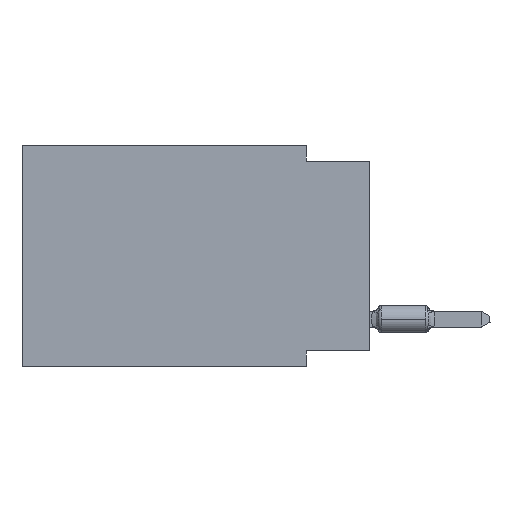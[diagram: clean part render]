
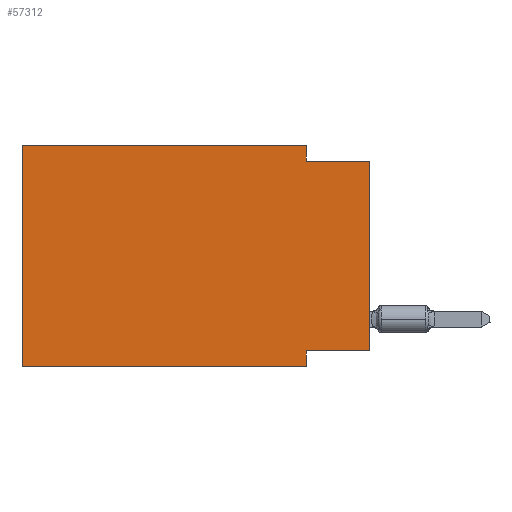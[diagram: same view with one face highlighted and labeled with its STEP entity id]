
A CAD part, left-side view. The second image highlights one B-rep face of the part: STEP entity #57312.
In plain terms, the highlighted planar face has unit normal (-1, 0, 0).
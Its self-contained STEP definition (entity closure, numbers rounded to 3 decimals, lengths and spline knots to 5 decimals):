
#2422 = EDGE_CURVE ( 'NONE', #3368, #60465, #82838, .T. ) ;
#3368 = VERTEX_POINT ( 'NONE', #6891 ) ;
#6891 = CARTESIAN_POINT ( 'NONE',  ( 0., 0.1, -0.325 ) ) ;
#7135 = ORIENTED_EDGE ( 'NONE', *, *, #54907, .F. ) ;
#7476 = DIRECTION ( 'NONE',  ( 0., -1., 0. ) ) ;
#9867 = CARTESIAN_POINT ( 'NONE',  ( 0., 0.55, 0. ) ) ;
#10330 = CARTESIAN_POINT ( 'NONE',  ( 0., 0.55, -0.35 ) ) ;
#13351 = ORIENTED_EDGE ( 'NONE', *, *, #19834, .F. ) ;
#15161 = CARTESIAN_POINT ( 'NONE',  ( 0., 0., -0.025 ) ) ;
#16466 = AXIS2_PLACEMENT_3D ( 'NONE', #69238, #44053, #76487 ) ;
#19517 = CARTESIAN_POINT ( 'NONE',  ( 0., 0.1, 0. ) ) ;
#19834 = EDGE_CURVE ( 'NONE', #46831, #79480, #67953, .T. ) ;
#19960 = LINE ( 'NONE', #65215, #42718 ) ;
#23024 = VERTEX_POINT ( 'NONE', #57015 ) ;
#23394 = ORIENTED_EDGE ( 'NONE', *, *, #31127, .T. ) ;
#23513 = DIRECTION ( 'NONE',  ( 0., 0., -1. ) ) ;
#25919 = LINE ( 'NONE', #19517, #65794 ) ;
#27560 = CARTESIAN_POINT ( 'NONE',  ( 0., 0.55, 0. ) ) ;
#30010 = ORIENTED_EDGE ( 'NONE', *, *, #72743, .F. ) ;
#30091 = VECTOR ( 'NONE', #64018, 39.37008 ) ;
#30718 = LINE ( 'NONE', #83676, #39320 ) ;
#31127 = EDGE_CURVE ( 'NONE', #59747, #60465, #19960, .T. ) ;
#31130 = DIRECTION ( 'NONE',  ( 0., 0., 1. ) ) ;
#34595 = CARTESIAN_POINT ( 'NONE',  ( 0., 0., -0.025 ) ) ;
#37839 = LINE ( 'NONE', #77131, #67518 ) ;
#39320 = VECTOR ( 'NONE', #31130, 39.37008 ) ;
#41335 = VERTEX_POINT ( 'NONE', #34595 ) ;
#42060 = CARTESIAN_POINT ( 'NONE',  ( 0., 0.1, 0. ) ) ;
#42187 = VERTEX_POINT ( 'NONE', #80932 ) ;
#42337 = DIRECTION ( 'NONE',  ( 0., -1., 0. ) ) ;
#42536 = EDGE_LOOP ( 'NONE', ( #52966, #64097, #65174, #13351, #7135, #23394, #67527, #30010 ) ) ;
#42718 = VECTOR ( 'NONE', #59651, 39.37008 ) ;
#43191 = FACE_OUTER_BOUND ( 'NONE', #42536, .T. ) ;
#43218 = EDGE_CURVE ( 'NONE', #79480, #42187, #25919, .T. ) ;
#44053 = DIRECTION ( 'NONE',  ( 1., 0., 0. ) ) ;
#44890 = VECTOR ( 'NONE', #23513, 39.37008 ) ;
#45086 = DIRECTION ( 'NONE',  ( 0., 1., 0. ) ) ;
#45553 = DIRECTION ( 'NONE',  ( 0., 0., -1. ) ) ;
#46340 = LINE ( 'NONE', #15161, #66051 ) ;
#46831 = VERTEX_POINT ( 'NONE', #27560 ) ;
#52966 = ORIENTED_EDGE ( 'NONE', *, *, #54688, .T. ) ;
#54688 = EDGE_CURVE ( 'NONE', #23024, #41335, #77694, .T. ) ;
#54907 = EDGE_CURVE ( 'NONE', #59747, #46831, #30718, .T. ) ;
#56626 = CARTESIAN_POINT ( 'NONE',  ( 0., 0.1, -0.35 ) ) ;
#57015 = CARTESIAN_POINT ( 'NONE',  ( 0., 0., -0.325 ) ) ;
#57312 = ADVANCED_FACE ( 'NONE', ( #43191 ), #63256, .F. ) ;
#59651 = DIRECTION ( 'NONE',  ( 0., -1., 0. ) ) ;
#59747 = VERTEX_POINT ( 'NONE', #10330 ) ;
#60465 = VERTEX_POINT ( 'NONE', #56626 ) ;
#63256 = PLANE ( 'NONE',  #16466 ) ;
#64018 = DIRECTION ( 'NONE',  ( 0., 0., 1. ) ) ;
#64097 = ORIENTED_EDGE ( 'NONE', *, *, #69961, .F. ) ;
#65174 = ORIENTED_EDGE ( 'NONE', *, *, #43218, .F. ) ;
#65215 = CARTESIAN_POINT ( 'NONE',  ( 0., 0.55, -0.35 ) ) ;
#65794 = VECTOR ( 'NONE', #45553, 39.37008 ) ;
#66051 = VECTOR ( 'NONE', #7476, 39.37008 ) ;
#67518 = VECTOR ( 'NONE', #45086, 39.37008 ) ;
#67527 = ORIENTED_EDGE ( 'NONE', *, *, #2422, .F. ) ;
#67953 = LINE ( 'NONE', #9867, #76754 ) ;
#69238 = CARTESIAN_POINT ( 'NONE',  ( 0., 0.55, 0. ) ) ;
#69961 = EDGE_CURVE ( 'NONE', #42187, #41335, #46340, .T. ) ;
#72743 = EDGE_CURVE ( 'NONE', #23024, #3368, #37839, .T. ) ;
#76487 = DIRECTION ( 'NONE',  ( 0., 0., -1. ) ) ;
#76754 = VECTOR ( 'NONE', #42337, 39.37008 ) ;
#77131 = CARTESIAN_POINT ( 'NONE',  ( 0., 0., -0.325 ) ) ;
#77262 = CARTESIAN_POINT ( 'NONE',  ( 0., 0., 0. ) ) ;
#77694 = LINE ( 'NONE', #77262, #30091 ) ;
#79480 = VERTEX_POINT ( 'NONE', #42060 ) ;
#80932 = CARTESIAN_POINT ( 'NONE',  ( 0., 0.1, -0.025 ) ) ;
#82421 = CARTESIAN_POINT ( 'NONE',  ( 0., 0.1, -0.35 ) ) ;
#82838 = LINE ( 'NONE', #82421, #44890 ) ;
#83676 = CARTESIAN_POINT ( 'NONE',  ( 0., 0.55, 0. ) ) ;
